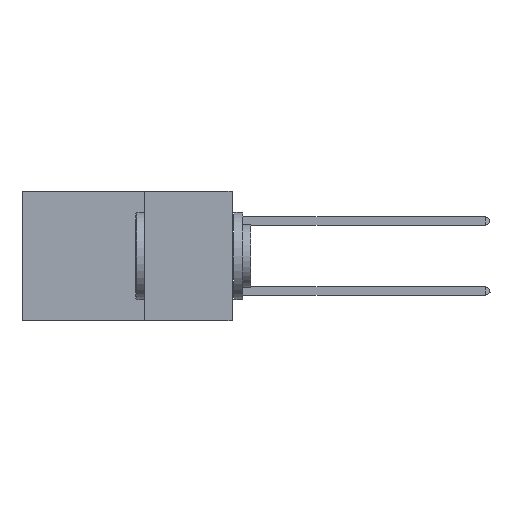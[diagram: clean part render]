
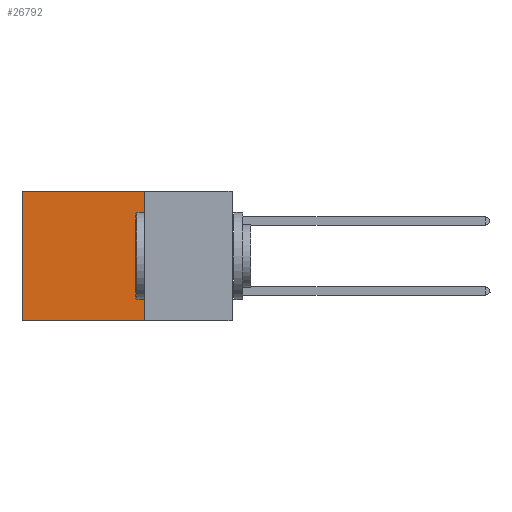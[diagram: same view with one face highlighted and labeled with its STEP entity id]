
A CAD part, left-side view. The second image highlights one B-rep face of the part: STEP entity #26792.
In plain terms, the highlighted planar face has unit normal (-1, 0, 0).
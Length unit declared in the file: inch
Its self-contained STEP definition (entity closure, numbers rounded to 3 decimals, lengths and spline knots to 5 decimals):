
#296 = CARTESIAN_POINT ( 'NONE',  ( 0.2875, 0.25, 0. ) ) ;
#4152 = CARTESIAN_POINT ( 'NONE',  ( 0.2875, 0.25, 0. ) ) ;
#5678 = VECTOR ( 'NONE', #29774, 39.37008 ) ;
#7690 = ORIENTED_EDGE ( 'NONE', *, *, #20063, .T. ) ;
#7713 = DIRECTION ( 'NONE',  ( 0., 1., 0. ) ) ;
#7761 = VERTEX_POINT ( 'NONE', #24052 ) ;
#8214 = AXIS2_PLACEMENT_3D ( 'NONE', #296, #15704, #9416 ) ;
#8356 = FACE_OUTER_BOUND ( 'NONE', #31314, .T. ) ;
#9416 = DIRECTION ( 'NONE',  ( 0., 0., -1. ) ) ;
#9477 = ORIENTED_EDGE ( 'NONE', *, *, #15277, .F. ) ;
#9552 = LINE ( 'NONE', #41088, #39552 ) ;
#11345 = CARTESIAN_POINT ( 'NONE',  ( 0.2875, 0.25, -0.37 ) ) ;
#12400 = DIRECTION ( 'NONE',  ( 0., 0., -1. ) ) ;
#12407 = DIRECTION ( 'NONE',  ( 0., 0., -1. ) ) ;
#14753 = VERTEX_POINT ( 'NONE', #17397 ) ;
#15277 = EDGE_CURVE ( 'NONE', #7761, #21793, #17133, .T. ) ;
#15704 = DIRECTION ( 'NONE',  ( 1., 0., 0. ) ) ;
#17133 = LINE ( 'NONE', #11345, #40661 ) ;
#17397 = CARTESIAN_POINT ( 'NONE',  ( 0.2875, 0.25, 0. ) ) ;
#17506 = CARTESIAN_POINT ( 'NONE',  ( 0.2875, 0.6, 0. ) ) ;
#18896 = EDGE_CURVE ( 'NONE', #14753, #7761, #35823, .T. ) ;
#20010 = ORIENTED_EDGE ( 'NONE', *, *, #18896, .F. ) ;
#20063 = EDGE_CURVE ( 'NONE', #14753, #34287, #20230, .T. ) ;
#20230 = LINE ( 'NONE', #4152, #5678 ) ;
#21793 = VERTEX_POINT ( 'NONE', #30251 ) ;
#22103 = CARTESIAN_POINT ( 'NONE',  ( 0.2875, 0.25, 0. ) ) ;
#24052 = CARTESIAN_POINT ( 'NONE',  ( 0.2875, 0.25, -0.37 ) ) ;
#25271 = PLANE ( 'NONE',  #8214 ) ;
#26792 = ADVANCED_FACE ( 'NONE', ( #8356 ), #25271, .F. ) ;
#27371 = VECTOR ( 'NONE', #12400, 39.37008 ) ;
#29774 = DIRECTION ( 'NONE',  ( 0., 1., 0. ) ) ;
#30251 = CARTESIAN_POINT ( 'NONE',  ( 0.2875, 0.6, -0.37 ) ) ;
#31314 = EDGE_LOOP ( 'NONE', ( #31782, #9477, #20010, #7690 ) ) ;
#31342 = EDGE_CURVE ( 'NONE', #34287, #21793, #9552, .T. ) ;
#31782 = ORIENTED_EDGE ( 'NONE', *, *, #31342, .T. ) ;
#34287 = VERTEX_POINT ( 'NONE', #17506 ) ;
#35823 = LINE ( 'NONE', #22103, #27371 ) ;
#39552 = VECTOR ( 'NONE', #12407, 39.37008 ) ;
#40661 = VECTOR ( 'NONE', #7713, 39.37008 ) ;
#41088 = CARTESIAN_POINT ( 'NONE',  ( 0.2875, 0.6, 0. ) ) ;
